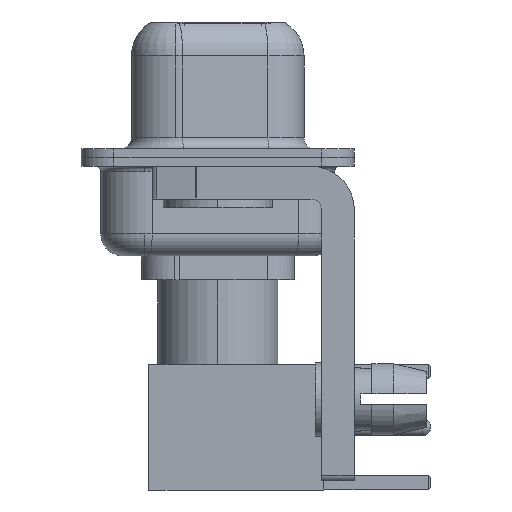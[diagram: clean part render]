
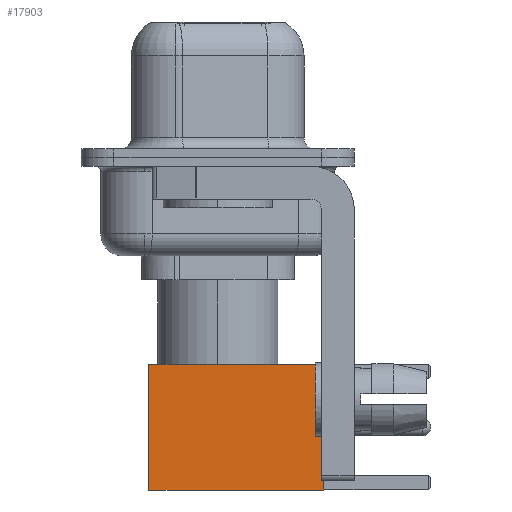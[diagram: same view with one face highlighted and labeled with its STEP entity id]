
A CAD part, left-side view. The second image highlights one B-rep face of the part: STEP entity #17903.
In plain terms, the highlighted face is planar.
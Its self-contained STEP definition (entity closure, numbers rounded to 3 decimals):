
#49 = EDGE_LOOP ( 'NONE', ( #9152, #17885, #5646, #15695 ) ) ;
#1692 = DIRECTION ( 'NONE',  ( 0., 0., -1. ) ) ;
#2128 = DIRECTION ( 'NONE',  ( -1., 0., 0. ) ) ;
#2805 = LINE ( 'NONE', #6042, #7732 ) ;
#2987 = CARTESIAN_POINT ( 'NONE',  ( -2.875, 2.875, 0. ) ) ;
#3001 = LINE ( 'NONE', #17447, #8336 ) ;
#3064 = CARTESIAN_POINT ( 'NONE',  ( 2.875, 2.875, 0. ) ) ;
#3070 = VECTOR ( 'NONE', #8840, 1000. ) ;
#5099 = VERTEX_POINT ( 'NONE', #18107 ) ;
#5646 = ORIENTED_EDGE ( 'NONE', *, *, #10859, .F. ) ;
#6042 = CARTESIAN_POINT ( 'NONE',  ( 2.875, 2.875, 0. ) ) ;
#6470 = VERTEX_POINT ( 'NONE', #13184 ) ;
#6989 = FACE_OUTER_BOUND ( 'NONE', #49, .T. ) ;
#7732 = VECTOR ( 'NONE', #1692, 1000. ) ;
#8336 = VECTOR ( 'NONE', #8759, 1000. ) ;
#8459 = LINE ( 'NONE', #8916, #10471 ) ;
#8735 = DIRECTION ( 'NONE',  ( 0., 0., 1. ) ) ;
#8759 = DIRECTION ( 'NONE',  ( -1., 0., 0. ) ) ;
#8840 = DIRECTION ( 'NONE',  ( 0., 0., -1. ) ) ;
#8916 = CARTESIAN_POINT ( 'NONE',  ( 0., 2.875, 0. ) ) ;
#9152 = ORIENTED_EDGE ( 'NONE', *, *, #12140, .T. ) ;
#9542 = EDGE_CURVE ( 'NONE', #5099, #6470, #3001, .T. ) ;
#9794 = CARTESIAN_POINT ( 'NONE',  ( -2.875, 2.875, 0. ) ) ;
#10471 = VECTOR ( 'NONE', #2128, 1000. ) ;
#10859 = EDGE_CURVE ( 'NONE', #6470, #11644, #15740, .T. ) ;
#11644 = VERTEX_POINT ( 'NONE', #9794 ) ;
#12140 = EDGE_CURVE ( 'NONE', #5099, #15486, #2805, .T. ) ;
#12871 = CARTESIAN_POINT ( 'NONE',  ( 2.875, 2.875, 0. ) ) ;
#12926 = PLANE ( 'NONE',  #16460 ) ;
#13184 = CARTESIAN_POINT ( 'NONE',  ( -2.875, 2.875, 8. ) ) ;
#14514 = DIRECTION ( 'NONE',  ( 0., 1., 0. ) ) ;
#15486 = VERTEX_POINT ( 'NONE', #12871 ) ;
#15695 = ORIENTED_EDGE ( 'NONE', *, *, #9542, .F. ) ;
#15740 = LINE ( 'NONE', #2987, #3070 ) ;
#16460 = AXIS2_PLACEMENT_3D ( 'NONE', #3064, #14514, #8735 ) ;
#16582 = EDGE_CURVE ( 'NONE', #15486, #11644, #8459, .T. ) ;
#17447 = CARTESIAN_POINT ( 'NONE',  ( 0., 2.875, 8. ) ) ;
#17885 = ORIENTED_EDGE ( 'NONE', *, *, #16582, .T. ) ;
#17903 = ADVANCED_FACE ( 'NONE', ( #6989 ), #12926, .T. ) ;
#18107 = CARTESIAN_POINT ( 'NONE',  ( 2.875, 2.875, 8. ) ) ;
